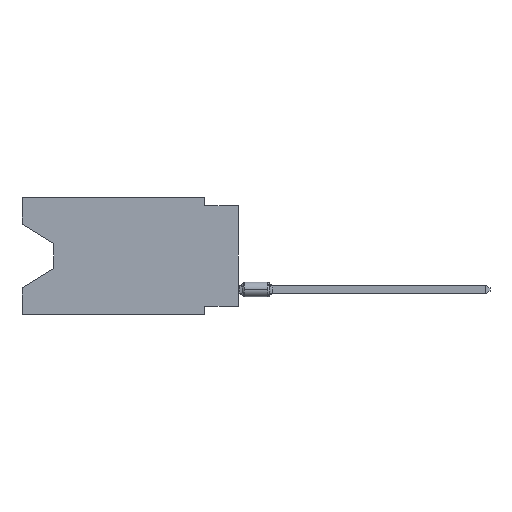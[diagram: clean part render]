
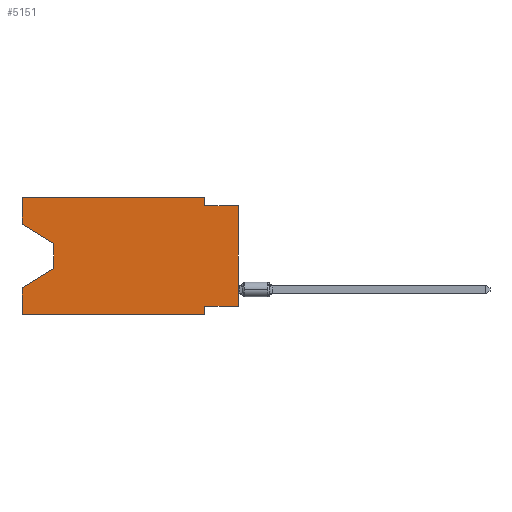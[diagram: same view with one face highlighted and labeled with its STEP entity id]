
A CAD part, left-side view. The second image highlights one B-rep face of the part: STEP entity #5151.
In plain terms, the highlighted planar face has unit normal (-1, 0, 0).
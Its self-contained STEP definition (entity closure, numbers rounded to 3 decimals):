
#109 = EDGE_LOOP ( 'NONE', ( #12694, #6619, #6055, #8335, #9561, #4224, #1930, #6525, #13296, #10045, #536, #7476 ) ) ;
#422 = LINE ( 'NONE', #731, #2722 ) ;
#496 = DIRECTION ( 'NONE',  ( 0., -1., 0. ) ) ;
#536 = ORIENTED_EDGE ( 'NONE', *, *, #10276, .F. ) ;
#731 = CARTESIAN_POINT ( 'NONE',  ( 0., 0., -0.635 ) ) ;
#799 = CARTESIAN_POINT ( 'NONE',  ( 0., 16.383, 0. ) ) ;
#1470 = DIRECTION ( 'NONE',  ( 0., 0., -1. ) ) ;
#1695 = EDGE_CURVE ( 'NONE', #7540, #9948, #6150, .T. ) ;
#1853 = VECTOR ( 'NONE', #7892, 1000. ) ;
#1919 = EDGE_CURVE ( 'NONE', #3122, #2624, #7556, .T. ) ;
#1930 = ORIENTED_EDGE ( 'NONE', *, *, #8584, .F. ) ;
#1961 = LINE ( 'NONE', #10135, #9050 ) ;
#1965 = VERTEX_POINT ( 'NONE', #6745 ) ;
#2097 = PLANE ( 'NONE',  #6655 ) ;
#2296 = VERTEX_POINT ( 'NONE', #3278 ) ;
#2420 = CARTESIAN_POINT ( 'NONE',  ( 0., 13.97, -3.505 ) ) ;
#2432 = VERTEX_POINT ( 'NONE', #2789 ) ;
#2624 = VERTEX_POINT ( 'NONE', #11273 ) ;
#2722 = VECTOR ( 'NONE', #12066, 1000. ) ;
#2789 = CARTESIAN_POINT ( 'NONE',  ( 0., 0., -0.635 ) ) ;
#3122 = VERTEX_POINT ( 'NONE', #8765 ) ;
#3130 = VECTOR ( 'NONE', #3480, 1000. ) ;
#3278 = CARTESIAN_POINT ( 'NONE',  ( 0., 2.54, 0. ) ) ;
#3480 = DIRECTION ( 'NONE',  ( 0., 1., 0. ) ) ;
#3745 = CARTESIAN_POINT ( 'NONE',  ( 0., 16.383, -8.89 ) ) ;
#4085 = LINE ( 'NONE', #8070, #8770 ) ;
#4224 = ORIENTED_EDGE ( 'NONE', *, *, #10073, .F. ) ;
#4375 = VECTOR ( 'NONE', #4527, 1000. ) ;
#4527 = DIRECTION ( 'NONE',  ( 0., 0., -1. ) ) ;
#4695 = CARTESIAN_POINT ( 'NONE',  ( 0., 16.383, 0. ) ) ;
#4890 = VERTEX_POINT ( 'NONE', #11620 ) ;
#4936 = DIRECTION ( 'NONE',  ( 0., 0., 1. ) ) ;
#4980 = CARTESIAN_POINT ( 'NONE',  ( 0., 16.383, -6.852 ) ) ;
#5151 = ADVANCED_FACE ( 'NONE', ( #6171 ), #2097, .F. ) ;
#5613 = LINE ( 'NONE', #12754, #10749 ) ;
#5671 = EDGE_CURVE ( 'NONE', #2296, #1965, #5613, .T. ) ;
#6055 = ORIENTED_EDGE ( 'NONE', *, *, #7805, .T. ) ;
#6150 = LINE ( 'NONE', #7155, #9955 ) ;
#6160 = DIRECTION ( 'NONE',  ( 0., 0.855, -0.519 ) ) ;
#6171 = FACE_OUTER_BOUND ( 'NONE', #109, .T. ) ;
#6292 = CARTESIAN_POINT ( 'NONE',  ( 0., 16.383, 0. ) ) ;
#6454 = CARTESIAN_POINT ( 'NONE',  ( 0., 16.383, -2.038 ) ) ;
#6525 = ORIENTED_EDGE ( 'NONE', *, *, #13182, .T. ) ;
#6619 = ORIENTED_EDGE ( 'NONE', *, *, #1919, .T. ) ;
#6655 = AXIS2_PLACEMENT_3D ( 'NONE', #6292, #10459, #11274 ) ;
#6745 = CARTESIAN_POINT ( 'NONE',  ( 0., 2.54, -0.635 ) ) ;
#7092 = VERTEX_POINT ( 'NONE', #13348 ) ;
#7155 = CARTESIAN_POINT ( 'NONE',  ( 0., 16.383, 0. ) ) ;
#7476 = ORIENTED_EDGE ( 'NONE', *, *, #1695, .F. ) ;
#7498 = EDGE_CURVE ( 'NONE', #12420, #4890, #10949, .T. ) ;
#7540 = VERTEX_POINT ( 'NONE', #6454 ) ;
#7556 = LINE ( 'NONE', #2420, #4375 ) ;
#7805 = EDGE_CURVE ( 'NONE', #2624, #12308, #12478, .T. ) ;
#7892 = DIRECTION ( 'NONE',  ( 0., -0.855, -0.519 ) ) ;
#8070 = CARTESIAN_POINT ( 'NONE',  ( 0., 2.54, -8.89 ) ) ;
#8222 = VECTOR ( 'NONE', #6160, 1000. ) ;
#8335 = ORIENTED_EDGE ( 'NONE', *, *, #10851, .F. ) ;
#8584 = EDGE_CURVE ( 'NONE', #7092, #11507, #10898, .T. ) ;
#8662 = LINE ( 'NONE', #4695, #11638 ) ;
#8765 = CARTESIAN_POINT ( 'NONE',  ( 0., 13.97, -3.505 ) ) ;
#8770 = VECTOR ( 'NONE', #9005, 1000. ) ;
#8818 = LINE ( 'NONE', #10915, #1853 ) ;
#9005 = DIRECTION ( 'NONE',  ( 0., 0., -1. ) ) ;
#9034 = EDGE_CURVE ( 'NONE', #1965, #2432, #422, .T. ) ;
#9050 = VECTOR ( 'NONE', #12223, 1000. ) ;
#9245 = CARTESIAN_POINT ( 'NONE',  ( 0., 13.97, -5.385 ) ) ;
#9365 = CARTESIAN_POINT ( 'NONE',  ( 0., 16.383, -8.89 ) ) ;
#9435 = EDGE_CURVE ( 'NONE', #7540, #3122, #8818, .T. ) ;
#9561 = ORIENTED_EDGE ( 'NONE', *, *, #7498, .T. ) ;
#9756 = CARTESIAN_POINT ( 'NONE',  ( 0., 0., -8.255 ) ) ;
#9920 = LINE ( 'NONE', #799, #11868 ) ;
#9948 = VERTEX_POINT ( 'NONE', #12724 ) ;
#9955 = VECTOR ( 'NONE', #10248, 1000. ) ;
#10045 = ORIENTED_EDGE ( 'NONE', *, *, #5671, .F. ) ;
#10073 = EDGE_CURVE ( 'NONE', #11507, #4890, #4085, .T. ) ;
#10135 = CARTESIAN_POINT ( 'NONE',  ( 0., 0., 0. ) ) ;
#10248 = DIRECTION ( 'NONE',  ( 0., 0., 1. ) ) ;
#10276 = EDGE_CURVE ( 'NONE', #9948, #2296, #8662, .T. ) ;
#10459 = DIRECTION ( 'NONE',  ( 1., 0., 0. ) ) ;
#10625 = DIRECTION ( 'NONE',  ( 0., -1., 0. ) ) ;
#10749 = VECTOR ( 'NONE', #1470, 1000. ) ;
#10803 = VECTOR ( 'NONE', #10625, 1000. ) ;
#10851 = EDGE_CURVE ( 'NONE', #12420, #12308, #9920, .T. ) ;
#10898 = LINE ( 'NONE', #9756, #3130 ) ;
#10915 = CARTESIAN_POINT ( 'NONE',  ( 0., 16.383, -2.038 ) ) ;
#10949 = LINE ( 'NONE', #3745, #10803 ) ;
#11273 = CARTESIAN_POINT ( 'NONE',  ( 0., 13.97, -5.385 ) ) ;
#11274 = DIRECTION ( 'NONE',  ( 0., 0., -1. ) ) ;
#11507 = VERTEX_POINT ( 'NONE', #11692 ) ;
#11620 = CARTESIAN_POINT ( 'NONE',  ( 0., 2.54, -8.89 ) ) ;
#11638 = VECTOR ( 'NONE', #496, 1000. ) ;
#11692 = CARTESIAN_POINT ( 'NONE',  ( 0., 2.54, -8.255 ) ) ;
#11868 = VECTOR ( 'NONE', #4936, 1000. ) ;
#12066 = DIRECTION ( 'NONE',  ( 0., -1., 0. ) ) ;
#12223 = DIRECTION ( 'NONE',  ( 0., 0., 1. ) ) ;
#12308 = VERTEX_POINT ( 'NONE', #4980 ) ;
#12420 = VERTEX_POINT ( 'NONE', #9365 ) ;
#12478 = LINE ( 'NONE', #9245, #8222 ) ;
#12694 = ORIENTED_EDGE ( 'NONE', *, *, #9435, .T. ) ;
#12724 = CARTESIAN_POINT ( 'NONE',  ( 0., 16.383, 0. ) ) ;
#12754 = CARTESIAN_POINT ( 'NONE',  ( 0., 2.54, 0. ) ) ;
#13182 = EDGE_CURVE ( 'NONE', #7092, #2432, #1961, .T. ) ;
#13296 = ORIENTED_EDGE ( 'NONE', *, *, #9034, .F. ) ;
#13348 = CARTESIAN_POINT ( 'NONE',  ( 0., 0., -8.255 ) ) ;
